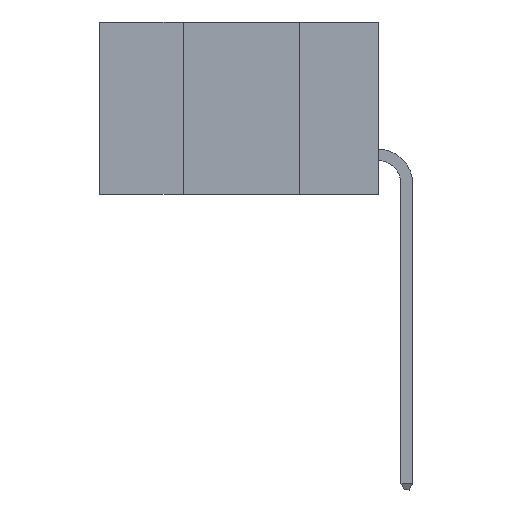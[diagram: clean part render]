
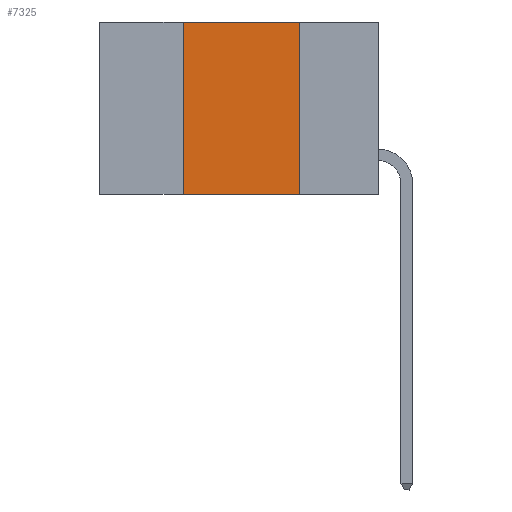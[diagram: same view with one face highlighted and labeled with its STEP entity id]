
A CAD part, left-side view. The second image highlights one B-rep face of the part: STEP entity #7325.
In plain terms, the highlighted planar face has unit normal (-1, 0, 0).
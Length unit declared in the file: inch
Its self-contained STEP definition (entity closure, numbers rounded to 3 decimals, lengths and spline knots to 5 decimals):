
#386 = CARTESIAN_POINT ( 'NONE',  ( 0., 0.42, -0.37 ) ) ;
#2031 = VERTEX_POINT ( 'NONE', #19386 ) ;
#2220 = DIRECTION ( 'NONE',  ( 0., -1., 0. ) ) ;
#2236 = CARTESIAN_POINT ( 'NONE',  ( 0., 0.42, 0. ) ) ;
#2427 = VECTOR ( 'NONE', #6057, 39.37008 ) ;
#3366 = VERTEX_POINT ( 'NONE', #10385 ) ;
#4434 = DIRECTION ( 'NONE',  ( 0., 0., -1. ) ) ;
#4438 = EDGE_CURVE ( 'NONE', #10992, #12180, #18355, .T. ) ;
#6057 = DIRECTION ( 'NONE',  ( 0., -1., 0. ) ) ;
#6104 = AXIS2_PLACEMENT_3D ( 'NONE', #13691, #15279, #8794 ) ;
#7325 = ADVANCED_FACE ( 'NONE', ( #19443 ), #13487, .F. ) ;
#7582 = ORIENTED_EDGE ( 'NONE', *, *, #15545, .F. ) ;
#8457 = ORIENTED_EDGE ( 'NONE', *, *, #4438, .F. ) ;
#8794 = DIRECTION ( 'NONE',  ( 0., 0., -1. ) ) ;
#9042 = ORIENTED_EDGE ( 'NONE', *, *, #20352, .T. ) ;
#9772 = LINE ( 'NONE', #12377, #14473 ) ;
#10385 = CARTESIAN_POINT ( 'NONE',  ( 0., 0.17, -0.37 ) ) ;
#10580 = VECTOR ( 'NONE', #2220, 39.37008 ) ;
#10949 = CARTESIAN_POINT ( 'NONE',  ( 0., 0.6, -0.37 ) ) ;
#10992 = VERTEX_POINT ( 'NONE', #386 ) ;
#12180 = VERTEX_POINT ( 'NONE', #15075 ) ;
#12377 = CARTESIAN_POINT ( 'NONE',  ( 0., 0.17, 0. ) ) ;
#12790 = LINE ( 'NONE', #19444, #10580 ) ;
#13001 = ORIENTED_EDGE ( 'NONE', *, *, #16550, .F. ) ;
#13487 = PLANE ( 'NONE',  #6104 ) ;
#13569 = LINE ( 'NONE', #10949, #2427 ) ;
#13691 = CARTESIAN_POINT ( 'NONE',  ( 0., 0.6, 0. ) ) ;
#14190 = VECTOR ( 'NONE', #16454, 39.37008 ) ;
#14473 = VECTOR ( 'NONE', #4434, 39.37008 ) ;
#15075 = CARTESIAN_POINT ( 'NONE',  ( 0., 0.42, 0. ) ) ;
#15279 = DIRECTION ( 'NONE',  ( 1., 0., 0. ) ) ;
#15545 = EDGE_CURVE ( 'NONE', #2031, #3366, #9772, .T. ) ;
#16454 = DIRECTION ( 'NONE',  ( 0., 0., 1. ) ) ;
#16550 = EDGE_CURVE ( 'NONE', #12180, #2031, #12790, .T. ) ;
#16667 = EDGE_LOOP ( 'NONE', ( #7582, #13001, #8457, #9042 ) ) ;
#18355 = LINE ( 'NONE', #2236, #14190 ) ;
#19386 = CARTESIAN_POINT ( 'NONE',  ( 0., 0.17, 0. ) ) ;
#19443 = FACE_OUTER_BOUND ( 'NONE', #16667, .T. ) ;
#19444 = CARTESIAN_POINT ( 'NONE',  ( 0., 0.6, 0. ) ) ;
#20352 = EDGE_CURVE ( 'NONE', #10992, #3366, #13569, .T. ) ;
